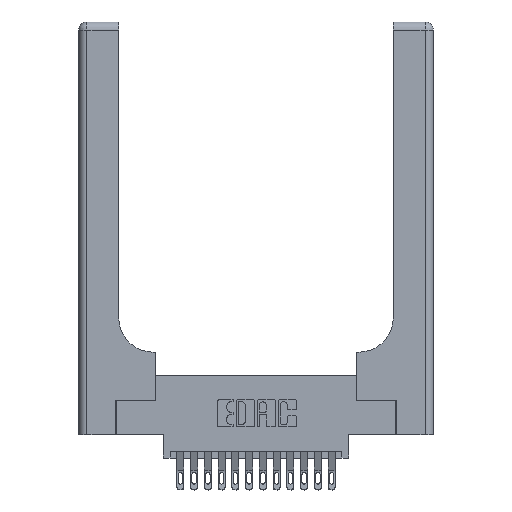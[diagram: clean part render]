
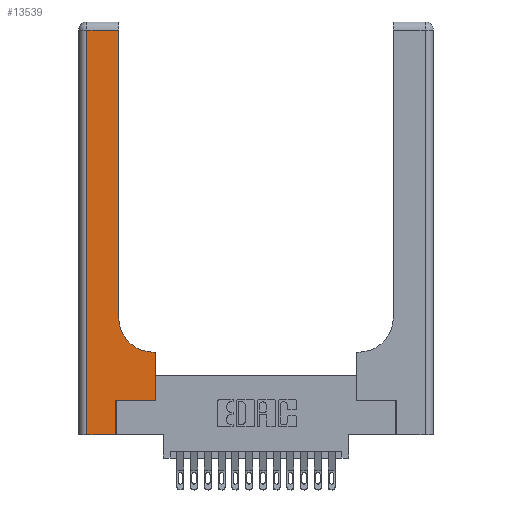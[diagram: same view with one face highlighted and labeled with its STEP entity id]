
A CAD part, top view. The second image highlights one B-rep face of the part: STEP entity #13539.
In plain terms, the highlighted planar face has unit normal (0, 0, 1).
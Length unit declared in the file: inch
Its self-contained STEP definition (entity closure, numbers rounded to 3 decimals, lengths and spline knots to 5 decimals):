
#142 = CARTESIAN_POINT ( 'NONE',  ( 0.06, 2.94, 0.37 ) ) ;
#455 = VERTEX_POINT ( 'NONE', #12107 ) ;
#868 = EDGE_CURVE ( 'NONE', #17386, #455, #10953, .T. ) ;
#949 = DIRECTION ( 'NONE',  ( 0., 1., 0. ) ) ;
#1061 = VECTOR ( 'NONE', #16854, 39.37008 ) ;
#1069 = LINE ( 'NONE', #15873, #8651 ) ;
#1097 = VERTEX_POINT ( 'NONE', #15194 ) ;
#1586 = CARTESIAN_POINT ( 'NONE',  ( 0.5415, 0.6, 0.37 ) ) ;
#2804 = ORIENTED_EDGE ( 'NONE', *, *, #3423, .T. ) ;
#3057 = VERTEX_POINT ( 'NONE', #1586 ) ;
#3149 = CARTESIAN_POINT ( 'NONE',  ( 0.269, 0.25, 0.37 ) ) ;
#3326 = VERTEX_POINT ( 'NONE', #17367 ) ;
#3423 = EDGE_CURVE ( 'NONE', #455, #4597, #3751, .T. ) ;
#3645 = DIRECTION ( 'NONE',  ( 0., 0., -1. ) ) ;
#3751 = LINE ( 'NONE', #17471, #6291 ) ;
#3835 = CARTESIAN_POINT ( 'NONE',  ( 0.06, 3., 0.37 ) ) ;
#3949 = DIRECTION ( 'NONE',  ( 0., 0., -1. ) ) ;
#4079 = DIRECTION ( 'NONE',  ( 0., 1., 0. ) ) ;
#4087 = LINE ( 'NONE', #18613, #7555 ) ;
#4177 = DIRECTION ( 'NONE',  ( -1., 0., 0. ) ) ;
#4497 = CARTESIAN_POINT ( 'NONE',  ( 0.2915, 0.85, 0.37 ) ) ;
#4597 = VERTEX_POINT ( 'NONE', #142 ) ;
#5362 = DIRECTION ( 'NONE',  ( 0., -1., 0. ) ) ;
#6080 = ORIENTED_EDGE ( 'NONE', *, *, #14454, .T. ) ;
#6291 = VECTOR ( 'NONE', #14373, 39.37008 ) ;
#6458 = DIRECTION ( 'NONE',  ( 1., 0., 0. ) ) ;
#6486 = VERTEX_POINT ( 'NONE', #12834 ) ;
#6710 = CARTESIAN_POINT ( 'NONE',  ( 0.5415, 0.85, 0.37 ) ) ;
#7439 = DIRECTION ( 'NONE',  ( 1., 0., 0. ) ) ;
#7555 = VECTOR ( 'NONE', #949, 39.37008 ) ;
#7674 = CIRCLE ( 'NONE', #10286, 0.25 ) ;
#7810 = LINE ( 'NONE', #14465, #11252 ) ;
#8160 = DIRECTION ( 'NONE',  ( -1., 0., 0. ) ) ;
#8271 = DIRECTION ( 'NONE',  ( 1., 0., 0. ) ) ;
#8340 = VECTOR ( 'NONE', #6458, 39.37008 ) ;
#8651 = VECTOR ( 'NONE', #4079, 39.37008 ) ;
#8785 = ORIENTED_EDGE ( 'NONE', *, *, #14009, .T. ) ;
#8823 = VERTEX_POINT ( 'NONE', #9049 ) ;
#9049 = CARTESIAN_POINT ( 'NONE',  ( 0.5585, 0.25, 0.37 ) ) ;
#9270 = ORIENTED_EDGE ( 'NONE', *, *, #868, .T. ) ;
#9626 = VERTEX_POINT ( 'NONE', #9866 ) ;
#9651 = ORIENTED_EDGE ( 'NONE', *, *, #12526, .T. ) ;
#9866 = CARTESIAN_POINT ( 'NONE',  ( 0.269, 0., 0.37 ) ) ;
#10286 = AXIS2_PLACEMENT_3D ( 'NONE', #6710, #3949, #8271 ) ;
#10513 = VECTOR ( 'NONE', #5362, 39.37008 ) ;
#10514 = ORIENTED_EDGE ( 'NONE', *, *, #14397, .T. ) ;
#10953 = LINE ( 'NONE', #12369, #1061 ) ;
#11214 = ORIENTED_EDGE ( 'NONE', *, *, #12443, .T. ) ;
#11252 = VECTOR ( 'NONE', #4177, 39.37008 ) ;
#11632 = ORIENTED_EDGE ( 'NONE', *, *, #18652, .T. ) ;
#12107 = CARTESIAN_POINT ( 'NONE',  ( 0.2915, 2.94, 0.37 ) ) ;
#12283 = LINE ( 'NONE', #18183, #8340 ) ;
#12369 = CARTESIAN_POINT ( 'NONE',  ( 0.2915, 3., 0.37 ) ) ;
#12443 = EDGE_CURVE ( 'NONE', #9626, #6486, #4087, .T. ) ;
#12526 = EDGE_CURVE ( 'NONE', #1097, #3057, #7810, .T. ) ;
#12834 = CARTESIAN_POINT ( 'NONE',  ( 0.269, 0.25, 0.37 ) ) ;
#13109 = AXIS2_PLACEMENT_3D ( 'NONE', #18388, #3645, #8160 ) ;
#13300 = LINE ( 'NONE', #3835, #10513 ) ;
#13437 = ORIENTED_EDGE ( 'NONE', *, *, #18728, .T. ) ;
#13539 = ADVANCED_FACE ( 'NONE', ( #13787 ), #15554, .F. ) ;
#13787 = FACE_OUTER_BOUND ( 'NONE', #18911, .T. ) ;
#14009 = EDGE_CURVE ( 'NONE', #6486, #8823, #15409, .T. ) ;
#14373 = DIRECTION ( 'NONE',  ( -1., 0., 0. ) ) ;
#14397 = EDGE_CURVE ( 'NONE', #4597, #3326, #13300, .T. ) ;
#14454 = EDGE_CURVE ( 'NONE', #8823, #1097, #1069, .T. ) ;
#14465 = CARTESIAN_POINT ( 'NONE',  ( 0.2915, 0.6, 0.37 ) ) ;
#15194 = CARTESIAN_POINT ( 'NONE',  ( 0.5585, 0.6, 0.37 ) ) ;
#15409 = LINE ( 'NONE', #3149, #18404 ) ;
#15554 = PLANE ( 'NONE',  #13109 ) ;
#15873 = CARTESIAN_POINT ( 'NONE',  ( 0.5585, 0.25, 0.37 ) ) ;
#16854 = DIRECTION ( 'NONE',  ( 0., 1., 0. ) ) ;
#17367 = CARTESIAN_POINT ( 'NONE',  ( 0.06, 0., 0.37 ) ) ;
#17386 = VERTEX_POINT ( 'NONE', #4497 ) ;
#17471 = CARTESIAN_POINT ( 'NONE',  ( 0., 2.94, 0.37 ) ) ;
#18183 = CARTESIAN_POINT ( 'NONE',  ( 0., 0., 0.37 ) ) ;
#18388 = CARTESIAN_POINT ( 'NONE',  ( 0., 3., 0.37 ) ) ;
#18404 = VECTOR ( 'NONE', #7439, 39.37008 ) ;
#18613 = CARTESIAN_POINT ( 'NONE',  ( 0.269, 0., 0.37 ) ) ;
#18652 = EDGE_CURVE ( 'NONE', #3326, #9626, #12283, .T. ) ;
#18728 = EDGE_CURVE ( 'NONE', #3057, #17386, #7674, .T. ) ;
#18911 = EDGE_LOOP ( 'NONE', ( #9270, #2804, #10514, #11632, #11214, #8785, #6080, #9651, #13437 ) ) ;
